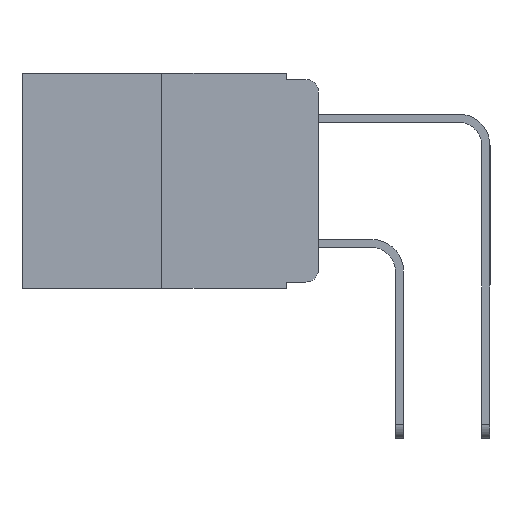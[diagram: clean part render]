
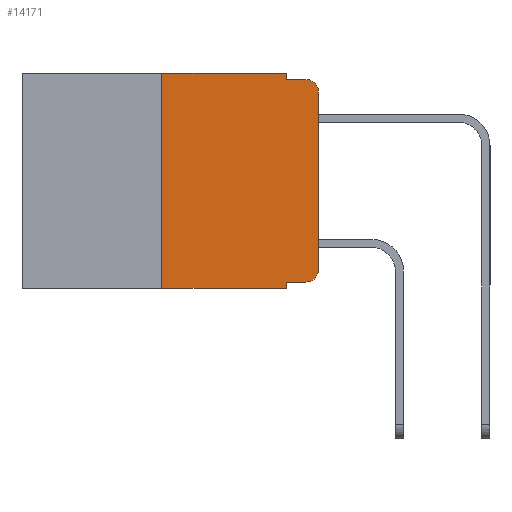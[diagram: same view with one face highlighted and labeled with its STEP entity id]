
A CAD part, left-side view. The second image highlights one B-rep face of the part: STEP entity #14171.
In plain terms, the highlighted planar face has unit normal (-1, 0, 0).
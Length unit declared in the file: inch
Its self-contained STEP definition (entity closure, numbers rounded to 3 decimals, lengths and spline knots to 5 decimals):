
#734 = CIRCLE ( 'NONE', #2814, 0.02 ) ;
#791 = CARTESIAN_POINT ( 'NONE',  ( 0., 0.02, -0.313 ) ) ;
#1011 = VERTEX_POINT ( 'NONE', #15115 ) ;
#1018 = CARTESIAN_POINT ( 'NONE',  ( 0., 0.02, -0.03 ) ) ;
#1319 = CIRCLE ( 'NONE', #13102, 0.02 ) ;
#1416 = DIRECTION ( 'NONE',  ( 0., 0., -1. ) ) ;
#1478 = ORIENTED_EDGE ( 'NONE', *, *, #7271, .F. ) ;
#1507 = CARTESIAN_POINT ( 'NONE',  ( 0., 0., -0.313 ) ) ;
#1782 = AXIS2_PLACEMENT_3D ( 'NONE', #15648, #5658, #14477 ) ;
#1830 = VERTEX_POINT ( 'NONE', #9848 ) ;
#2074 = LINE ( 'NONE', #15196, #8676 ) ;
#2203 = DIRECTION ( 'NONE',  ( 0., 0., -1. ) ) ;
#2276 = VECTOR ( 'NONE', #8243, 39.37008 ) ;
#2568 = EDGE_LOOP ( 'NONE', ( #14536, #8361, #1478, #8544, #8928, #15465, #9324, #15857, #12982, #3185 ) ) ;
#2597 = VECTOR ( 'NONE', #8542, 39.37008 ) ;
#2640 = VECTOR ( 'NONE', #16666, 39.37008 ) ;
#2739 = CARTESIAN_POINT ( 'NONE',  ( 0., 0.051, -0.343 ) ) ;
#2814 = AXIS2_PLACEMENT_3D ( 'NONE', #791, #10027, #2203 ) ;
#3160 = LINE ( 'NONE', #16043, #3573 ) ;
#3185 = ORIENTED_EDGE ( 'NONE', *, *, #15586, .T. ) ;
#3573 = VECTOR ( 'NONE', #12395, 39.37008 ) ;
#3817 = CARTESIAN_POINT ( 'NONE',  ( 0., 0.051, -0.01 ) ) ;
#3958 = EDGE_CURVE ( 'NONE', #1830, #13201, #12308, .T. ) ;
#4596 = EDGE_CURVE ( 'NONE', #9882, #8631, #12865, .T. ) ;
#4673 = DIRECTION ( 'NONE',  ( 0., -1., 0. ) ) ;
#4829 = LINE ( 'NONE', #3817, #11674 ) ;
#5326 = DIRECTION ( 'NONE',  ( 0., -1., 0. ) ) ;
#5485 = DIRECTION ( 'NONE',  ( 0., 0., 1. ) ) ;
#5560 = VECTOR ( 'NONE', #5326, 39.37008 ) ;
#5570 = CARTESIAN_POINT ( 'NONE',  ( 0., 0.051, -0.333 ) ) ;
#5658 = DIRECTION ( 'NONE',  ( 1., 0., 0. ) ) ;
#5733 = VECTOR ( 'NONE', #5485, 39.37008 ) ;
#6135 = CARTESIAN_POINT ( 'NONE',  ( 0., 0.473, 0. ) ) ;
#6375 = EDGE_CURVE ( 'NONE', #8631, #1011, #1319, .T. ) ;
#7218 = CARTESIAN_POINT ( 'NONE',  ( 0., 0.051, 0. ) ) ;
#7271 = EDGE_CURVE ( 'NONE', #8027, #1011, #4829, .T. ) ;
#7596 = DIRECTION ( 'NONE',  ( -1., 0., 0. ) ) ;
#7928 = EDGE_CURVE ( 'NONE', #12940, #15248, #2074, .T. ) ;
#8027 = VERTEX_POINT ( 'NONE', #10495 ) ;
#8153 = EDGE_CURVE ( 'NONE', #13201, #8027, #15416, .T. ) ;
#8243 = DIRECTION ( 'NONE',  ( 0., 0., -1. ) ) ;
#8361 = ORIENTED_EDGE ( 'NONE', *, *, #6375, .T. ) ;
#8542 = DIRECTION ( 'NONE',  ( 0., 0., -1. ) ) ;
#8544 = ORIENTED_EDGE ( 'NONE', *, *, #8153, .F. ) ;
#8631 = VERTEX_POINT ( 'NONE', #12884 ) ;
#8676 = VECTOR ( 'NONE', #9076, 39.37008 ) ;
#8928 = ORIENTED_EDGE ( 'NONE', *, *, #3958, .F. ) ;
#9076 = DIRECTION ( 'NONE',  ( 0., -1., 0. ) ) ;
#9324 = ORIENTED_EDGE ( 'NONE', *, *, #7928, .T. ) ;
#9840 = EDGE_CURVE ( 'NONE', #12940, #1830, #15736, .T. ) ;
#9848 = CARTESIAN_POINT ( 'NONE',  ( 0., 0.25, 0. ) ) ;
#9882 = VERTEX_POINT ( 'NONE', #1507 ) ;
#10027 = DIRECTION ( 'NONE',  ( -1., 0., 0. ) ) ;
#10495 = CARTESIAN_POINT ( 'NONE',  ( 0., 0.051, -0.01 ) ) ;
#10665 = EDGE_CURVE ( 'NONE', #11677, #15248, #15705, .T. ) ;
#10744 = CARTESIAN_POINT ( 'NONE',  ( 0., 0.25, -0.343 ) ) ;
#11674 = VECTOR ( 'NONE', #4673, 39.37008 ) ;
#11677 = VERTEX_POINT ( 'NONE', #5570 ) ;
#11793 = CARTESIAN_POINT ( 'NONE',  ( 0., 0.25, 0. ) ) ;
#12008 = PLANE ( 'NONE',  #1782 ) ;
#12308 = LINE ( 'NONE', #6135, #5560 ) ;
#12395 = DIRECTION ( 'NONE',  ( 0., -1., 0. ) ) ;
#12865 = LINE ( 'NONE', #15926, #2640 ) ;
#12884 = CARTESIAN_POINT ( 'NONE',  ( 0., 0., -0.03 ) ) ;
#12940 = VERTEX_POINT ( 'NONE', #10744 ) ;
#12982 = ORIENTED_EDGE ( 'NONE', *, *, #13119, .T. ) ;
#13102 = AXIS2_PLACEMENT_3D ( 'NONE', #1018, #7596, #1416 ) ;
#13119 = EDGE_CURVE ( 'NONE', #11677, #14454, #3160, .T. ) ;
#13201 = VERTEX_POINT ( 'NONE', #15945 ) ;
#13204 = CARTESIAN_POINT ( 'NONE',  ( 0., 0.051, 0. ) ) ;
#14171 = ADVANCED_FACE ( 'NONE', ( #16197 ), #12008, .F. ) ;
#14454 = VERTEX_POINT ( 'NONE', #16232 ) ;
#14477 = DIRECTION ( 'NONE',  ( 0., 0., -1. ) ) ;
#14536 = ORIENTED_EDGE ( 'NONE', *, *, #4596, .T. ) ;
#15115 = CARTESIAN_POINT ( 'NONE',  ( 0., 0.02, -0.01 ) ) ;
#15196 = CARTESIAN_POINT ( 'NONE',  ( 0., 0.473, -0.343 ) ) ;
#15248 = VERTEX_POINT ( 'NONE', #2739 ) ;
#15416 = LINE ( 'NONE', #13204, #2276 ) ;
#15465 = ORIENTED_EDGE ( 'NONE', *, *, #9840, .F. ) ;
#15586 = EDGE_CURVE ( 'NONE', #14454, #9882, #734, .T. ) ;
#15648 = CARTESIAN_POINT ( 'NONE',  ( 0., 0.473, 0. ) ) ;
#15705 = LINE ( 'NONE', #7218, #2597 ) ;
#15736 = LINE ( 'NONE', #11793, #5733 ) ;
#15857 = ORIENTED_EDGE ( 'NONE', *, *, #10665, .F. ) ;
#15926 = CARTESIAN_POINT ( 'NONE',  ( 0., 0., 0. ) ) ;
#15945 = CARTESIAN_POINT ( 'NONE',  ( 0., 0.051, 0. ) ) ;
#16043 = CARTESIAN_POINT ( 'NONE',  ( 0., 0.051, -0.333 ) ) ;
#16197 = FACE_OUTER_BOUND ( 'NONE', #2568, .T. ) ;
#16232 = CARTESIAN_POINT ( 'NONE',  ( 0., 0.02, -0.333 ) ) ;
#16666 = DIRECTION ( 'NONE',  ( 0., 0., 1. ) ) ;
